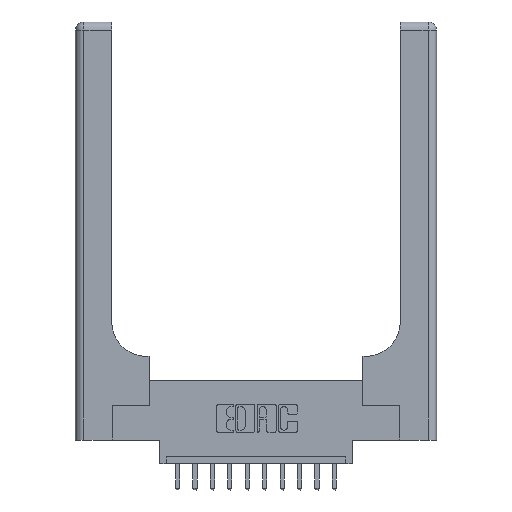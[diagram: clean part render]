
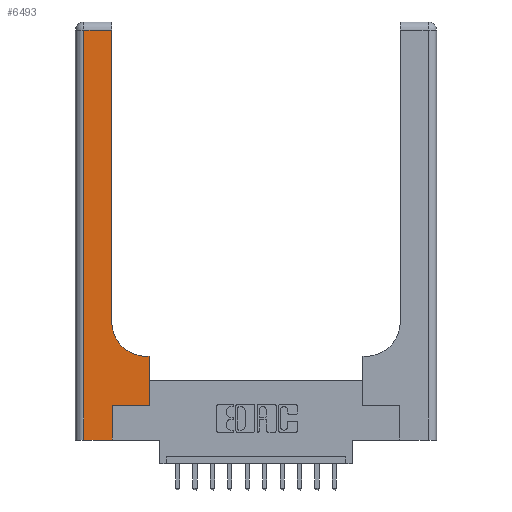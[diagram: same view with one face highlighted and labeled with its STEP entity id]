
A CAD part, top view. The second image highlights one B-rep face of the part: STEP entity #6493.
In plain terms, the highlighted planar face has unit normal (0, 0, 1).
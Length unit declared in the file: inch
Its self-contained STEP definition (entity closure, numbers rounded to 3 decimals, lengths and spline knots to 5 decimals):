
#82 = VECTOR ( 'NONE', #4961, 39.37008 ) ;
#264 = VERTEX_POINT ( 'NONE', #14548 ) ;
#612 = VERTEX_POINT ( 'NONE', #2139 ) ;
#617 = CARTESIAN_POINT ( 'NONE',  ( 0.265, 0., 0.37 ) ) ;
#774 = LINE ( 'NONE', #10917, #3720 ) ;
#863 = DIRECTION ( 'NONE',  ( -1., 0., 0. ) ) ;
#898 = VERTEX_POINT ( 'NONE', #617 ) ;
#919 = LINE ( 'NONE', #16257, #9233 ) ;
#1277 = CARTESIAN_POINT ( 'NONE',  ( 0.26, 0.85, 0.37 ) ) ;
#1458 = EDGE_CURVE ( 'NONE', #5275, #264, #2492, .T. ) ;
#2025 = ORIENTED_EDGE ( 'NONE', *, *, #5354, .T. ) ;
#2139 = CARTESIAN_POINT ( 'NONE',  ( 0.528, 0.6, 0.37 ) ) ;
#2492 = LINE ( 'NONE', #7563, #4288 ) ;
#2662 = LINE ( 'NONE', #5139, #4285 ) ;
#2780 = VECTOR ( 'NONE', #5737, 39.37008 ) ;
#2912 = ORIENTED_EDGE ( 'NONE', *, *, #15855, .T. ) ;
#3462 = CARTESIAN_POINT ( 'NONE',  ( 0.528, 0.25, 0.37 ) ) ;
#3720 = VECTOR ( 'NONE', #863, 39.37008 ) ;
#3920 = DIRECTION ( 'NONE',  ( 1., 0., 0. ) ) ;
#4285 = VECTOR ( 'NONE', #10218, 39.37008 ) ;
#4288 = VECTOR ( 'NONE', #13726, 39.37008 ) ;
#4321 = CARTESIAN_POINT ( 'NONE',  ( 0., 3., 0.37 ) ) ;
#4565 = LINE ( 'NONE', #12239, #8035 ) ;
#4803 = ORIENTED_EDGE ( 'NONE', *, *, #1458, .T. ) ;
#4873 = CIRCLE ( 'NONE', #14184, 0.25 ) ;
#4895 = CARTESIAN_POINT ( 'NONE',  ( 0.06, 3., 0.37 ) ) ;
#4961 = DIRECTION ( 'NONE',  ( 0., 1., 0. ) ) ;
#5139 = CARTESIAN_POINT ( 'NONE',  ( 0.265, 0.25, 0.37 ) ) ;
#5180 = CARTESIAN_POINT ( 'NONE',  ( 0.265, 0.25, 0.37 ) ) ;
#5275 = VERTEX_POINT ( 'NONE', #1277 ) ;
#5354 = EDGE_CURVE ( 'NONE', #612, #11134, #5492, .T. ) ;
#5492 = LINE ( 'NONE', #10566, #2780 ) ;
#5581 = FACE_OUTER_BOUND ( 'NONE', #9356, .T. ) ;
#5737 = DIRECTION ( 'NONE',  ( -1., 0., 0. ) ) ;
#6493 = ADVANCED_FACE ( 'NONE', ( #5581 ), #10656, .F. ) ;
#6603 = ORIENTED_EDGE ( 'NONE', *, *, #10528, .T. ) ;
#6797 = EDGE_CURVE ( 'NONE', #14198, #12637, #2662, .T. ) ;
#7054 = CARTESIAN_POINT ( 'NONE',  ( 0.528, 0.25, 0.37 ) ) ;
#7459 = EDGE_CURVE ( 'NONE', #11134, #5275, #4873, .T. ) ;
#7563 = CARTESIAN_POINT ( 'NONE',  ( 0.26, 3., 0.37 ) ) ;
#7648 = DIRECTION ( 'NONE',  ( 0., -1., 0. ) ) ;
#7951 = VECTOR ( 'NONE', #7648, 39.37008 ) ;
#8035 = VECTOR ( 'NONE', #11160, 39.37008 ) ;
#8167 = EDGE_CURVE ( 'NONE', #898, #14198, #919, .T. ) ;
#8783 = CARTESIAN_POINT ( 'NONE',  ( 0.51, 0.85, 0.37 ) ) ;
#9233 = VECTOR ( 'NONE', #12470, 39.37008 ) ;
#9356 = EDGE_LOOP ( 'NONE', ( #4803, #15489, #15715, #6603, #15043, #10374, #2912, #2025, #14526 ) ) ;
#9412 = DIRECTION ( 'NONE',  ( -1., 0., 0. ) ) ;
#9486 = DIRECTION ( 'NONE',  ( 0., 0., -1. ) ) ;
#10218 = DIRECTION ( 'NONE',  ( 1., 0., 0. ) ) ;
#10374 = ORIENTED_EDGE ( 'NONE', *, *, #6797, .T. ) ;
#10528 = EDGE_CURVE ( 'NONE', #14022, #898, #4565, .T. ) ;
#10566 = CARTESIAN_POINT ( 'NONE',  ( 0.26, 0.6, 0.37 ) ) ;
#10656 = PLANE ( 'NONE',  #13680 ) ;
#10917 = CARTESIAN_POINT ( 'NONE',  ( 0., 2.94, 0.37 ) ) ;
#11134 = VERTEX_POINT ( 'NONE', #13283 ) ;
#11160 = DIRECTION ( 'NONE',  ( 1., 0., 0. ) ) ;
#12239 = CARTESIAN_POINT ( 'NONE',  ( 0., 0., 0.37 ) ) ;
#12461 = EDGE_CURVE ( 'NONE', #13005, #14022, #13905, .T. ) ;
#12470 = DIRECTION ( 'NONE',  ( 0., 1., 0. ) ) ;
#12637 = VERTEX_POINT ( 'NONE', #7054 ) ;
#12767 = DIRECTION ( 'NONE',  ( 0., 0., -1. ) ) ;
#13005 = VERTEX_POINT ( 'NONE', #15162 ) ;
#13283 = CARTESIAN_POINT ( 'NONE',  ( 0.51, 0.6, 0.37 ) ) ;
#13680 = AXIS2_PLACEMENT_3D ( 'NONE', #4321, #9486, #9412 ) ;
#13726 = DIRECTION ( 'NONE',  ( 0., 1., 0. ) ) ;
#13905 = LINE ( 'NONE', #4895, #7951 ) ;
#14022 = VERTEX_POINT ( 'NONE', #14836 ) ;
#14184 = AXIS2_PLACEMENT_3D ( 'NONE', #8783, #12767, #3920 ) ;
#14198 = VERTEX_POINT ( 'NONE', #5180 ) ;
#14526 = ORIENTED_EDGE ( 'NONE', *, *, #7459, .T. ) ;
#14548 = CARTESIAN_POINT ( 'NONE',  ( 0.26, 2.94, 0.37 ) ) ;
#14836 = CARTESIAN_POINT ( 'NONE',  ( 0.06, 0., 0.37 ) ) ;
#14947 = EDGE_CURVE ( 'NONE', #264, #13005, #774, .T. ) ;
#15043 = ORIENTED_EDGE ( 'NONE', *, *, #8167, .T. ) ;
#15102 = LINE ( 'NONE', #3462, #82 ) ;
#15162 = CARTESIAN_POINT ( 'NONE',  ( 0.06, 2.94, 0.37 ) ) ;
#15489 = ORIENTED_EDGE ( 'NONE', *, *, #14947, .T. ) ;
#15715 = ORIENTED_EDGE ( 'NONE', *, *, #12461, .T. ) ;
#15855 = EDGE_CURVE ( 'NONE', #12637, #612, #15102, .T. ) ;
#16257 = CARTESIAN_POINT ( 'NONE',  ( 0.265, 0., 0.37 ) ) ;
